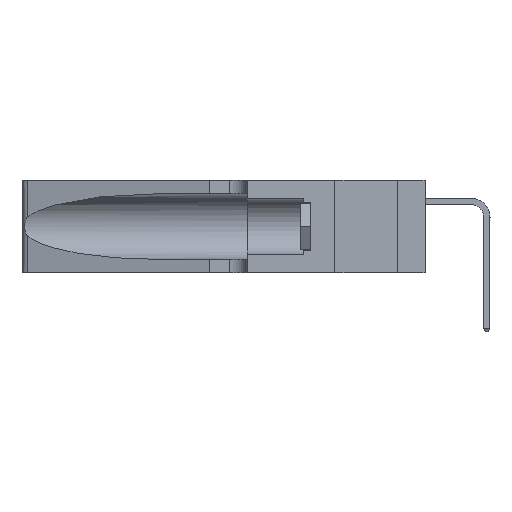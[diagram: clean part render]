
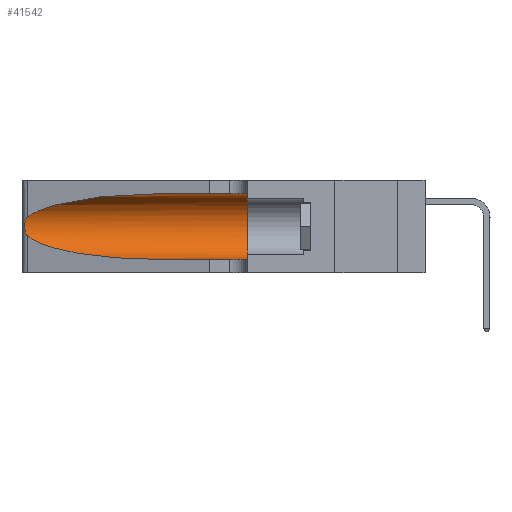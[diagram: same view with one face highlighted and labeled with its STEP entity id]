
A CAD part, left-side view. The second image highlights one B-rep face of the part: STEP entity #41542.
In plain terms, the highlighted cylindrical face has radius 3.308 mm (diameter 6.617 mm), a partial arc.
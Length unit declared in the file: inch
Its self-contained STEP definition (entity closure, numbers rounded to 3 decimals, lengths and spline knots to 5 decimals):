
#76 = AXIS2_PLACEMENT_3D ( 'NONE', #22556, #880, #26217 ) ;
#235 = VERTEX_POINT ( 'NONE', #11265 ) ;
#690 = ORIENTED_EDGE ( 'NONE', *, *, #46112, .T. ) ;
#784 = CARTESIAN_POINT ( 'NONE',  ( 0.25487, 1.22718, 0.14631 ) ) ;
#880 = DIRECTION ( 'NONE',  ( 0., -1., 0. ) ) ;
#1859 = CARTESIAN_POINT ( 'NONE',  ( 0.1305, 1.61858, 0.31525 ) ) ;
#2020 = CARTESIAN_POINT ( 'NONE',  ( 0.1305, 0.72297, 0.31525 ) ) ;
#2657 = EDGE_CURVE ( 'NONE', #22778, #235, #4490, .T. ) ;
#2963 = ORIENTED_EDGE ( 'NONE', *, *, #43923, .T. ) ;
#4226 = CARTESIAN_POINT ( 'NONE',  ( 0.25787, 1.23484, 0.2124 ) ) ;
#4490 = CIRCLE ( 'NONE', #22598, 0.13025 ) ;
#5831 = ORIENTED_EDGE ( 'NONE', *, *, #2657, .F. ) ;
#6169 = LINE ( 'NONE', #1859, #24287 ) ;
#6269 =( BOUNDED_CURVE ( )  B_SPLINE_CURVE ( 3, ( #33101, #32949, #40382, #18618 ),
 .UNSPECIFIED., .F., .F. ) 
 B_SPLINE_CURVE_WITH_KNOTS ( ( 4, 4 ),
 ( 1.5708, 2.84003 ),
 .UNSPECIFIED. ) 
 CURVE ( )  GEOMETRIC_REPRESENTATION_ITEM ( )  RATIONAL_B_SPLINE_CURVE ( ( 1., 0.87, 0.87, 1. ) ) 
 REPRESENTATION_ITEM ( '' )  );
#7896 = CARTESIAN_POINT ( 'NONE',  ( 0.26018, 1.23835, 0.19895 ) ) ;
#11265 = CARTESIAN_POINT ( 'NONE',  ( 0.1305, 0.35, 0.05475 ) ) ;
#11477 = CARTESIAN_POINT ( 'NONE',  ( 0.25487, 1.22718, 0.22369 ) ) ;
#11506 = CARTESIAN_POINT ( 'NONE',  ( 0.26075, 1.23896, 0.178 ) ) ;
#11894 = VERTEX_POINT ( 'NONE', #46493 ) ;
#12755 = DIRECTION ( 'NONE',  ( 0., -1., 0. ) ) ;
#14374 = CARTESIAN_POINT ( 'NONE',  ( 0.25555, 1.22994, 0.2215 ) ) ;
#14719 = CARTESIAN_POINT ( 'NONE',  ( 0.1305, 0.35, 0.185 ) ) ;
#15176 = CARTESIAN_POINT ( 'NONE',  ( 0.25856, 1.23593, 0.16098 ) ) ;
#15190 = CARTESIAN_POINT ( 'NONE',  ( 0.2373, 1.15595, 0.08982 ) ) ;
#15999 = ORIENTED_EDGE ( 'NONE', *, *, #33040, .T. ) ;
#17535 = CARTESIAN_POINT ( 'NONE',  ( 0.1305, 1.61858, 0.05475 ) ) ;
#18341 = DIRECTION ( 'NONE',  ( 0., 0., 1. ) ) ;
#18618 = CARTESIAN_POINT ( 'NONE',  ( 0.25487, 1.22718, 0.22369 ) ) ;
#18798 = CARTESIAN_POINT ( 'NONE',  ( 0.25639, 1.23186, 0.15144 ) ) ;
#18845 = ORIENTED_EDGE ( 'NONE', *, *, #44142, .F. ) ;
#18965 = CARTESIAN_POINT ( 'NONE',  ( 0.18966, 0.96281, 0.05475 ) ) ;
#21143 =( BOUNDED_CURVE ( )  B_SPLINE_CURVE ( 3, ( #784, #15190, #18965, #44389 ),
 .UNSPECIFIED., .F., .F. ) 
 B_SPLINE_CURVE_WITH_KNOTS ( ( 4, 4 ),
 ( 3.44316, 4.71239 ),
 .UNSPECIFIED. ) 
 CURVE ( )  GEOMETRIC_REPRESENTATION_ITEM ( )  RATIONAL_B_SPLINE_CURVE ( ( 1., 0.87, 0.87, 1. ) ) 
 REPRESENTATION_ITEM ( '' )  );
#22431 = CARTESIAN_POINT ( 'NONE',  ( 0.25487, 1.22718, 0.14631 ) ) ;
#22434 = CARTESIAN_POINT ( 'NONE',  ( 0.1305, 0.35, 0.31525 ) ) ;
#22556 = CARTESIAN_POINT ( 'NONE',  ( 0.1305, 1.61858, 0.185 ) ) ;
#22598 = AXIS2_PLACEMENT_3D ( 'NONE', #14719, #40122, #18341 ) ;
#22778 = VERTEX_POINT ( 'NONE', #22434 ) ;
#23004 = VERTEX_POINT ( 'NONE', #2020 ) ;
#23088 = B_SPLINE_CURVE_WITH_KNOTS ( 'NONE', 3,
 ( #39789, #14374, #25940, #4226, #29627, #7896, #33286, #11506, #36943, #15176, #40571, #18798, #44222, #22431 ),
 .UNSPECIFIED., .F., .F.,
 ( 4, 2, 2, 2, 2, 2, 4 ),
 ( 0., 0.00027, 0.00053, 0.00107, 0.0016, 0.00187, 0.00214 ),
 .UNSPECIFIED. ) ;
#23196 = CARTESIAN_POINT ( 'NONE',  ( 0.25487, 1.22718, 0.14631 ) ) ;
#23403 = CYLINDRICAL_SURFACE ( 'NONE', #76, 0.13025 ) ;
#23947 = ORIENTED_EDGE ( 'NONE', *, *, #41278, .T. ) ;
#24287 = VECTOR ( 'NONE', #12755, 39.37008 ) ;
#24809 = DIRECTION ( 'NONE',  ( 0., -1., 0. ) ) ;
#25940 = CARTESIAN_POINT ( 'NONE',  ( 0.25639, 1.23184, 0.21858 ) ) ;
#26217 = DIRECTION ( 'NONE',  ( 0., 0., -1. ) ) ;
#26279 = LINE ( 'NONE', #17535, #44480 ) ;
#29627 = CARTESIAN_POINT ( 'NONE',  ( 0.25854, 1.2359, 0.20912 ) ) ;
#31643 = VERTEX_POINT ( 'NONE', #11477 ) ;
#32949 = CARTESIAN_POINT ( 'NONE',  ( 0.18966, 0.96281, 0.31525 ) ) ;
#33040 = EDGE_CURVE ( 'NONE', #39753, #11894, #21143, .T. ) ;
#33101 = CARTESIAN_POINT ( 'NONE',  ( 0.1305, 0.72297, 0.31525 ) ) ;
#33286 = CARTESIAN_POINT ( 'NONE',  ( 0.26075, 1.23896, 0.19203 ) ) ;
#36873 = EDGE_LOOP ( 'NONE', ( #690, #2963, #15999, #23947, #5831, #18845 ) ) ;
#36943 = CARTESIAN_POINT ( 'NONE',  ( 0.26017, 1.23833, 0.17102 ) ) ;
#39753 = VERTEX_POINT ( 'NONE', #23196 ) ;
#39789 = CARTESIAN_POINT ( 'NONE',  ( 0.25487, 1.22718, 0.22369 ) ) ;
#40122 = DIRECTION ( 'NONE',  ( 0., 1., 0. ) ) ;
#40382 = CARTESIAN_POINT ( 'NONE',  ( 0.2373, 1.15595, 0.28018 ) ) ;
#40571 = CARTESIAN_POINT ( 'NONE',  ( 0.25789, 1.23486, 0.15765 ) ) ;
#41278 = EDGE_CURVE ( 'NONE', #11894, #235, #26279, .T. ) ;
#41542 = ADVANCED_FACE ( 'NONE', ( #42752 ), #23403, .F. ) ;
#42752 = FACE_OUTER_BOUND ( 'NONE', #36873, .T. ) ;
#43923 = EDGE_CURVE ( 'NONE', #31643, #39753, #23088, .T. ) ;
#44142 = EDGE_CURVE ( 'NONE', #23004, #22778, #6169, .T. ) ;
#44222 = CARTESIAN_POINT ( 'NONE',  ( 0.25555, 1.22993, 0.14849 ) ) ;
#44389 = CARTESIAN_POINT ( 'NONE',  ( 0.1305, 0.72297, 0.05475 ) ) ;
#44480 = VECTOR ( 'NONE', #24809, 39.37008 ) ;
#46112 = EDGE_CURVE ( 'NONE', #23004, #31643, #6269, .T. ) ;
#46493 = CARTESIAN_POINT ( 'NONE',  ( 0.1305, 0.72297, 0.05475 ) ) ;
